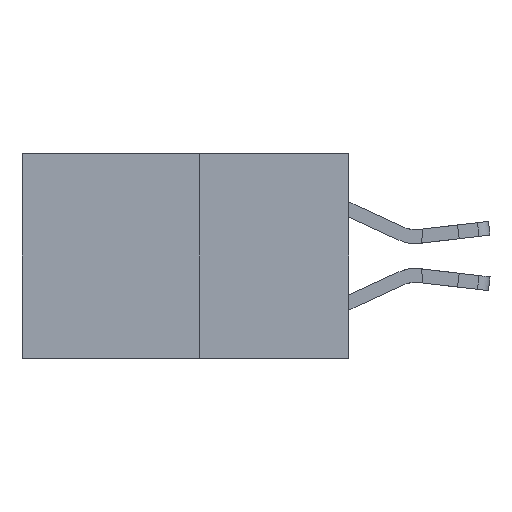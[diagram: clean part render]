
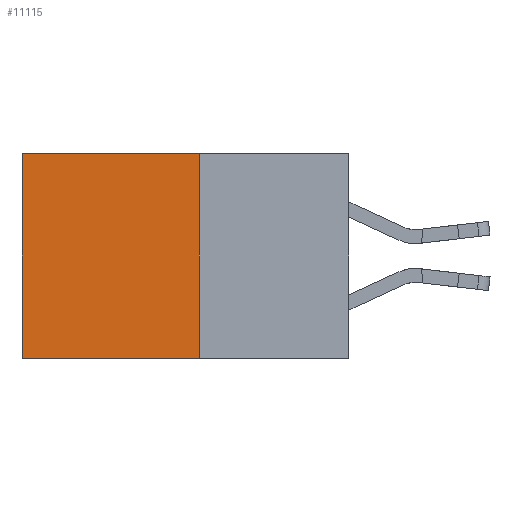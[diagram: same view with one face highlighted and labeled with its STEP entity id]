
A CAD part, left-side view. The second image highlights one B-rep face of the part: STEP entity #11115.
In plain terms, the highlighted planar face has unit normal (-1, 0, 0).
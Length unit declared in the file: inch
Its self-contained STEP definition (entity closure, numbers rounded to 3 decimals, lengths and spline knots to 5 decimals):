
#472 = EDGE_LOOP ( 'NONE', ( #1150, #15838, #13412, #3517 ) ) ;
#498 = CARTESIAN_POINT ( 'NONE',  ( 0.277, 0.27, 0. ) ) ;
#1150 = ORIENTED_EDGE ( 'NONE', *, *, #11184, .T. ) ;
#1703 = AXIS2_PLACEMENT_3D ( 'NONE', #12864, #5494, #14122 ) ;
#2038 = VECTOR ( 'NONE', #5238, 39.37008 ) ;
#2109 = FACE_OUTER_BOUND ( 'NONE', #472, .T. ) ;
#2173 = LINE ( 'NONE', #6677, #8283 ) ;
#3048 = PLANE ( 'NONE',  #1703 ) ;
#3179 = CARTESIAN_POINT ( 'NONE',  ( 0.277, 0.59, 0. ) ) ;
#3517 = ORIENTED_EDGE ( 'NONE', *, *, #4332, .T. ) ;
#3733 = CARTESIAN_POINT ( 'NONE',  ( 0.277, 0.59, -0.37 ) ) ;
#4332 = EDGE_CURVE ( 'NONE', #12925, #9502, #9403, .T. ) ;
#5185 = CARTESIAN_POINT ( 'NONE',  ( 0.277, 0.27, -0.37 ) ) ;
#5238 = DIRECTION ( 'NONE',  ( 0., 1., 0. ) ) ;
#5494 = DIRECTION ( 'NONE',  ( 1., 0., 0. ) ) ;
#6677 = CARTESIAN_POINT ( 'NONE',  ( 0.277, 0.27, -0.37 ) ) ;
#7871 = DIRECTION ( 'NONE',  ( 0., 0., -1. ) ) ;
#8053 = CARTESIAN_POINT ( 'NONE',  ( 0.277, 0.59, -0.37 ) ) ;
#8283 = VECTOR ( 'NONE', #7871, 39.37008 ) ;
#8692 = EDGE_CURVE ( 'NONE', #12925, #12011, #2173, .T. ) ;
#9403 = LINE ( 'NONE', #12604, #12316 ) ;
#9502 = VERTEX_POINT ( 'NONE', #3179 ) ;
#10727 = VECTOR ( 'NONE', #12984, 39.37008 ) ;
#11039 = LINE ( 'NONE', #5185, #2038 ) ;
#11115 = ADVANCED_FACE ( 'NONE', ( #2109 ), #3048, .F. ) ;
#11184 = EDGE_CURVE ( 'NONE', #9502, #14015, #11513, .T. ) ;
#11513 = LINE ( 'NONE', #8053, #10727 ) ;
#12011 = VERTEX_POINT ( 'NONE', #13231 ) ;
#12021 = DIRECTION ( 'NONE',  ( 0., 1., 0. ) ) ;
#12316 = VECTOR ( 'NONE', #12021, 39.37008 ) ;
#12604 = CARTESIAN_POINT ( 'NONE',  ( 0.277, 0.27, 0. ) ) ;
#12864 = CARTESIAN_POINT ( 'NONE',  ( 0.277, 0.27, -0.37 ) ) ;
#12925 = VERTEX_POINT ( 'NONE', #498 ) ;
#12984 = DIRECTION ( 'NONE',  ( 0., 0., -1. ) ) ;
#13231 = CARTESIAN_POINT ( 'NONE',  ( 0.277, 0.27, -0.37 ) ) ;
#13412 = ORIENTED_EDGE ( 'NONE', *, *, #8692, .F. ) ;
#13488 = EDGE_CURVE ( 'NONE', #12011, #14015, #11039, .T. ) ;
#14015 = VERTEX_POINT ( 'NONE', #3733 ) ;
#14122 = DIRECTION ( 'NONE',  ( 0., 0., -1. ) ) ;
#15838 = ORIENTED_EDGE ( 'NONE', *, *, #13488, .F. ) ;
